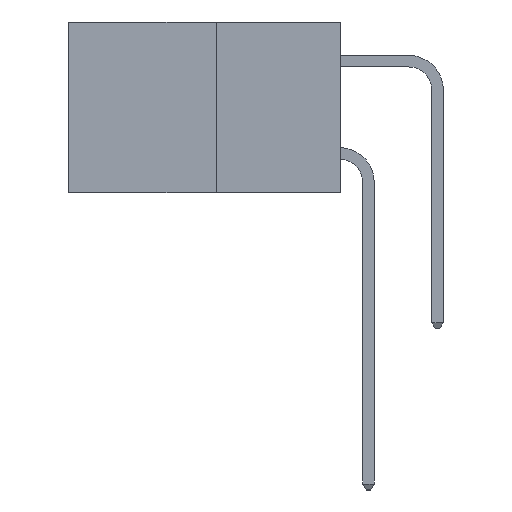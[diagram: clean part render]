
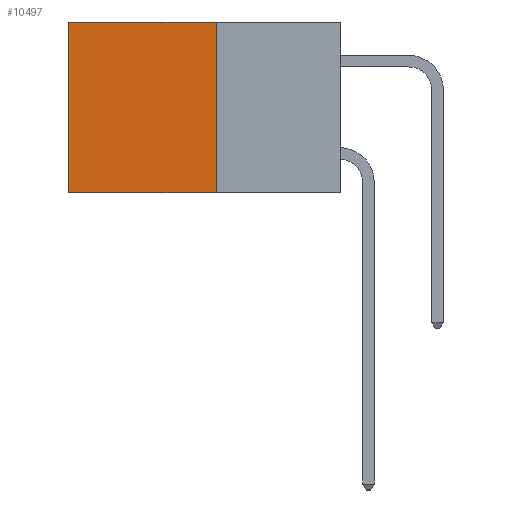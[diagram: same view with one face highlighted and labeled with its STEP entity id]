
A CAD part, left-side view. The second image highlights one B-rep face of the part: STEP entity #10497.
In plain terms, the highlighted planar face has unit normal (-1, 0, 0).
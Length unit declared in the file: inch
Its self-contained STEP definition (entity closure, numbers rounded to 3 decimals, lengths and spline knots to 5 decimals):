
#474 = DIRECTION ( 'NONE',  ( 0., 0., -1. ) ) ;
#1086 = DIRECTION ( 'NONE',  ( 0., 1., 0. ) ) ;
#1179 = CARTESIAN_POINT ( 'NONE',  ( 0.277, 0.59, -0.37 ) ) ;
#1576 = EDGE_CURVE ( 'NONE', #5574, #6271, #4106, .T. ) ;
#2695 = EDGE_CURVE ( 'NONE', #6356, #6271, #3925, .T. ) ;
#2856 = CARTESIAN_POINT ( 'NONE',  ( 0.277, 0.27, 0. ) ) ;
#3355 = DIRECTION ( 'NONE',  ( 0., 0., -1. ) ) ;
#3411 = CARTESIAN_POINT ( 'NONE',  ( 0.277, 0.27, -0.37 ) ) ;
#3722 = VERTEX_POINT ( 'NONE', #2856 ) ;
#3874 = CARTESIAN_POINT ( 'NONE',  ( 0.277, 0.59, -0.37 ) ) ;
#3925 = LINE ( 'NONE', #11746, #11557 ) ;
#4106 = LINE ( 'NONE', #1179, #11724 ) ;
#4433 = FACE_OUTER_BOUND ( 'NONE', #10370, .T. ) ;
#4582 = AXIS2_PLACEMENT_3D ( 'NONE', #10501, #6487, #474 ) ;
#5574 = VERTEX_POINT ( 'NONE', #8928 ) ;
#5628 = LINE ( 'NONE', #8268, #8053 ) ;
#5678 = EDGE_CURVE ( 'NONE', #3722, #6356, #5628, .T. ) ;
#6271 = VERTEX_POINT ( 'NONE', #3874 ) ;
#6356 = VERTEX_POINT ( 'NONE', #3411 ) ;
#6487 = DIRECTION ( 'NONE',  ( 1., 0., 0. ) ) ;
#6591 = VECTOR ( 'NONE', #1086, 39.37008 ) ;
#7287 = EDGE_CURVE ( 'NONE', #3722, #5574, #9296, .T. ) ;
#7598 = ORIENTED_EDGE ( 'NONE', *, *, #1576, .T. ) ;
#8053 = VECTOR ( 'NONE', #8249, 39.37008 ) ;
#8249 = DIRECTION ( 'NONE',  ( 0., 0., -1. ) ) ;
#8268 = CARTESIAN_POINT ( 'NONE',  ( 0.277, 0.27, -0.37 ) ) ;
#8928 = CARTESIAN_POINT ( 'NONE',  ( 0.277, 0.59, 0. ) ) ;
#9178 = ORIENTED_EDGE ( 'NONE', *, *, #7287, .T. ) ;
#9238 = ORIENTED_EDGE ( 'NONE', *, *, #5678, .F. ) ;
#9296 = LINE ( 'NONE', #12745, #6591 ) ;
#9482 = ORIENTED_EDGE ( 'NONE', *, *, #2695, .F. ) ;
#10370 = EDGE_LOOP ( 'NONE', ( #7598, #9482, #9238, #9178 ) ) ;
#10497 = ADVANCED_FACE ( 'NONE', ( #4433 ), #12274, .F. ) ;
#10501 = CARTESIAN_POINT ( 'NONE',  ( 0.277, 0.27, -0.37 ) ) ;
#11557 = VECTOR ( 'NONE', #12456, 39.37008 ) ;
#11724 = VECTOR ( 'NONE', #3355, 39.37008 ) ;
#11746 = CARTESIAN_POINT ( 'NONE',  ( 0.277, 0.27, -0.37 ) ) ;
#12274 = PLANE ( 'NONE',  #4582 ) ;
#12456 = DIRECTION ( 'NONE',  ( 0., 1., 0. ) ) ;
#12745 = CARTESIAN_POINT ( 'NONE',  ( 0.277, 0.27, 0. ) ) ;
